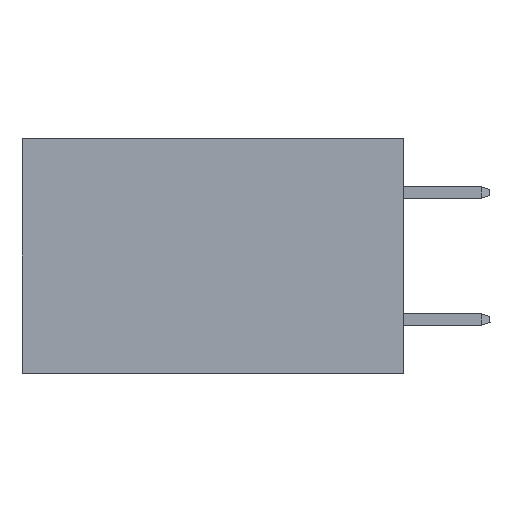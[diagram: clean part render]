
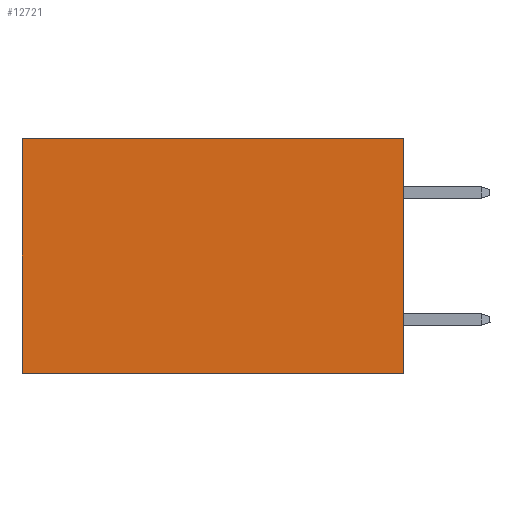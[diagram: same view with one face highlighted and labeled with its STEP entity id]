
A CAD part, left-side view. The second image highlights one B-rep face of the part: STEP entity #12721.
In plain terms, the highlighted planar face has unit normal (-1, 0, 0).
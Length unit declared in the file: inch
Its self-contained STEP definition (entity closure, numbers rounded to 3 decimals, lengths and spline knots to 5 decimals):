
#13 = DIRECTION ( 'NONE',  ( 0., 0., -1. ) ) ;
#103 = EDGE_CURVE ( 'NONE', #3758, #9595, #7412, .T. ) ;
#781 = AXIS2_PLACEMENT_3D ( 'NONE', #4659, #4486, #16571 ) ;
#1306 = CARTESIAN_POINT ( 'NONE',  ( 0.2875, 0., 0. ) ) ;
#1806 = CARTESIAN_POINT ( 'NONE',  ( 0.2875, 0., -0.37 ) ) ;
#3163 = EDGE_CURVE ( 'NONE', #3758, #13675, #11928, .T. ) ;
#3520 = PLANE ( 'NONE',  #781 ) ;
#3758 = VERTEX_POINT ( 'NONE', #8437 ) ;
#3888 = VECTOR ( 'NONE', #5884, 39.37008 ) ;
#4382 = CARTESIAN_POINT ( 'NONE',  ( 0.2875, 0.6, 0. ) ) ;
#4486 = DIRECTION ( 'NONE',  ( 1., 0., 0. ) ) ;
#4659 = CARTESIAN_POINT ( 'NONE',  ( 0.2875, 0., 0. ) ) ;
#4699 = DIRECTION ( 'NONE',  ( 0., 1., 0. ) ) ;
#4812 = CARTESIAN_POINT ( 'NONE',  ( 0.2875, 0., -0.37 ) ) ;
#4890 = ORIENTED_EDGE ( 'NONE', *, *, #3163, .F. ) ;
#5215 = ORIENTED_EDGE ( 'NONE', *, *, #9035, .F. ) ;
#5279 = VECTOR ( 'NONE', #4699, 39.37008 ) ;
#5294 = EDGE_CURVE ( 'NONE', #9595, #10574, #15262, .T. ) ;
#5731 = LINE ( 'NONE', #1806, #5905 ) ;
#5884 = DIRECTION ( 'NONE',  ( 0., 0., -1. ) ) ;
#5894 = VECTOR ( 'NONE', #13, 39.37008 ) ;
#5905 = VECTOR ( 'NONE', #12252, 39.37008 ) ;
#5981 = CARTESIAN_POINT ( 'NONE',  ( 0.2875, 0.6, 0. ) ) ;
#7126 = EDGE_LOOP ( 'NONE', ( #9261, #5215, #4890, #8388 ) ) ;
#7412 = LINE ( 'NONE', #12547, #5279 ) ;
#8388 = ORIENTED_EDGE ( 'NONE', *, *, #103, .T. ) ;
#8437 = CARTESIAN_POINT ( 'NONE',  ( 0.2875, 0., 0. ) ) ;
#9035 = EDGE_CURVE ( 'NONE', #13675, #10574, #5731, .T. ) ;
#9261 = ORIENTED_EDGE ( 'NONE', *, *, #5294, .T. ) ;
#9595 = VERTEX_POINT ( 'NONE', #5981 ) ;
#10574 = VERTEX_POINT ( 'NONE', #14512 ) ;
#11928 = LINE ( 'NONE', #1306, #5894 ) ;
#12252 = DIRECTION ( 'NONE',  ( 0., 1., 0. ) ) ;
#12547 = CARTESIAN_POINT ( 'NONE',  ( 0.2875, 0., 0. ) ) ;
#12721 = ADVANCED_FACE ( 'NONE', ( #15188 ), #3520, .F. ) ;
#13675 = VERTEX_POINT ( 'NONE', #4812 ) ;
#14512 = CARTESIAN_POINT ( 'NONE',  ( 0.2875, 0.6, -0.37 ) ) ;
#15188 = FACE_OUTER_BOUND ( 'NONE', #7126, .T. ) ;
#15262 = LINE ( 'NONE', #4382, #3888 ) ;
#16571 = DIRECTION ( 'NONE',  ( 0., 0., -1. ) ) ;
